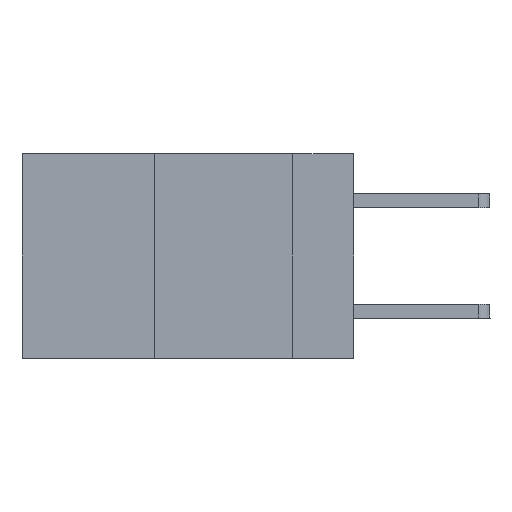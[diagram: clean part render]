
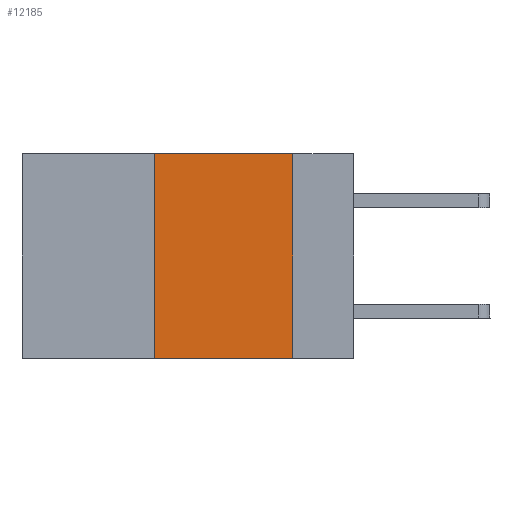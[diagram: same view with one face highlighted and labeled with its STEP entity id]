
A CAD part, left-side view. The second image highlights one B-rep face of the part: STEP entity #12185.
In plain terms, the highlighted planar face has unit normal (-1, 0, 0).
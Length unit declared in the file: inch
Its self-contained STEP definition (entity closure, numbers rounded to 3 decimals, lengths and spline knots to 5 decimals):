
#391 = VECTOR ( 'NONE', #6739, 39.37008 ) ;
#657 = EDGE_CURVE ( 'NONE', #7881, #6768, #816, .T. ) ;
#816 = LINE ( 'NONE', #8106, #391 ) ;
#1066 = DIRECTION ( 'NONE',  ( 0., 0., 1. ) ) ;
#1708 = LINE ( 'NONE', #14131, #9519 ) ;
#2007 = ORIENTED_EDGE ( 'NONE', *, *, #9537, .F. ) ;
#2801 = VECTOR ( 'NONE', #1066, 39.37008 ) ;
#2934 = VECTOR ( 'NONE', #9444, 39.37008 ) ;
#3005 = DIRECTION ( 'NONE',  ( 0., 0., -1. ) ) ;
#3134 = FACE_OUTER_BOUND ( 'NONE', #8491, .T. ) ;
#3327 = CARTESIAN_POINT ( 'NONE',  ( 0., 0.36, 0. ) ) ;
#4355 = CARTESIAN_POINT ( 'NONE',  ( 0., 0.6, 0. ) ) ;
#4356 = CARTESIAN_POINT ( 'NONE',  ( 0., 0.36, -0.37 ) ) ;
#4446 = EDGE_CURVE ( 'NONE', #15628, #6768, #1708, .T. ) ;
#4535 = ORIENTED_EDGE ( 'NONE', *, *, #7120, .F. ) ;
#4871 = CARTESIAN_POINT ( 'NONE',  ( 0., 0.36, 0. ) ) ;
#4888 = CARTESIAN_POINT ( 'NONE',  ( 0., 0.11, -0.37 ) ) ;
#6715 = DIRECTION ( 'NONE',  ( 0., 0., -1. ) ) ;
#6739 = DIRECTION ( 'NONE',  ( 0., -1., 0. ) ) ;
#6768 = VERTEX_POINT ( 'NONE', #4888 ) ;
#7120 = EDGE_CURVE ( 'NONE', #7881, #8349, #12203, .T. ) ;
#7881 = VERTEX_POINT ( 'NONE', #4356 ) ;
#8106 = CARTESIAN_POINT ( 'NONE',  ( 0., 0.6, -0.37 ) ) ;
#8138 = ORIENTED_EDGE ( 'NONE', *, *, #657, .T. ) ;
#8349 = VERTEX_POINT ( 'NONE', #3327 ) ;
#8491 = EDGE_LOOP ( 'NONE', ( #14224, #2007, #4535, #8138 ) ) ;
#9444 = DIRECTION ( 'NONE',  ( 0., -1., 0. ) ) ;
#9519 = VECTOR ( 'NONE', #3005, 39.37008 ) ;
#9537 = EDGE_CURVE ( 'NONE', #8349, #15628, #11982, .T. ) ;
#11583 = DIRECTION ( 'NONE',  ( 1., 0., 0. ) ) ;
#11982 = LINE ( 'NONE', #13036, #2934 ) ;
#12093 = CARTESIAN_POINT ( 'NONE',  ( 0., 0.11, 0. ) ) ;
#12185 = ADVANCED_FACE ( 'NONE', ( #3134 ), #12800, .F. ) ;
#12203 = LINE ( 'NONE', #4871, #2801 ) ;
#12800 = PLANE ( 'NONE',  #13622 ) ;
#13036 = CARTESIAN_POINT ( 'NONE',  ( 0., 0.6, 0. ) ) ;
#13622 = AXIS2_PLACEMENT_3D ( 'NONE', #4355, #11583, #6715 ) ;
#14131 = CARTESIAN_POINT ( 'NONE',  ( 0., 0.11, 0. ) ) ;
#14224 = ORIENTED_EDGE ( 'NONE', *, *, #4446, .F. ) ;
#15628 = VERTEX_POINT ( 'NONE', #12093 ) ;
